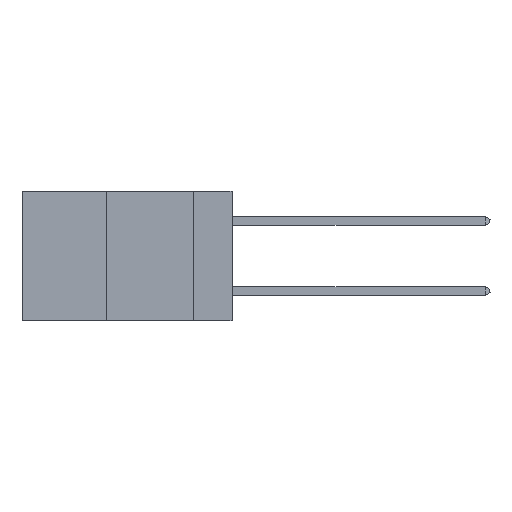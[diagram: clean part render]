
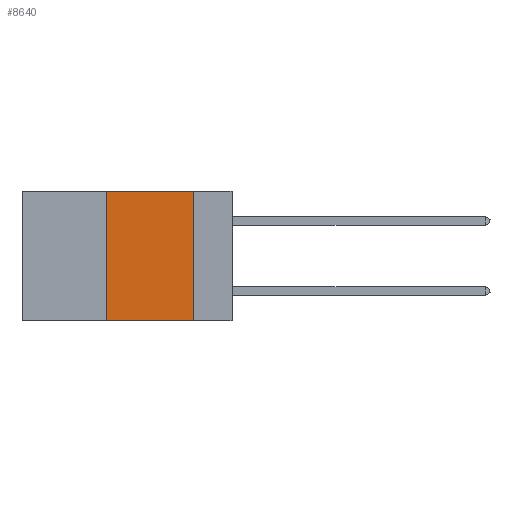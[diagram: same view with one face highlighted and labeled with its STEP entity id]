
A CAD part, left-side view. The second image highlights one B-rep face of the part: STEP entity #8640.
In plain terms, the highlighted planar face has unit normal (-1, 0, 0).
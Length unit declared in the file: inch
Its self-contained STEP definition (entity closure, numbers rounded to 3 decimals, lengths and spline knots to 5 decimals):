
#1943 = FACE_OUTER_BOUND ( 'NONE', #2229, .T. ) ;
#2229 = EDGE_LOOP ( 'NONE', ( #39148, #40176, #15780, #28841 ) ) ;
#3651 = LINE ( 'NONE', #20212, #40150 ) ;
#5818 = DIRECTION ( 'NONE',  ( 0., 0., -1. ) ) ;
#5874 = LINE ( 'NONE', #18531, #33836 ) ;
#6734 = EDGE_CURVE ( 'NONE', #27551, #7271, #3651, .T. ) ;
#7271 = VERTEX_POINT ( 'NONE', #43667 ) ;
#7871 = VECTOR ( 'NONE', #42710, 39.37008 ) ;
#8640 = ADVANCED_FACE ( 'NONE', ( #1943 ), #13028, .F. ) ;
#9150 = DIRECTION ( 'NONE',  ( 0., -1., 0. ) ) ;
#9687 = EDGE_CURVE ( 'NONE', #7271, #20230, #5874, .T. ) ;
#12099 = CARTESIAN_POINT ( 'NONE',  ( 0., 0.36, 0. ) ) ;
#13028 = PLANE ( 'NONE',  #21847 ) ;
#15780 = ORIENTED_EDGE ( 'NONE', *, *, #26651, .F. ) ;
#17183 = CARTESIAN_POINT ( 'NONE',  ( 0., 0.6, 0. ) ) ;
#18148 = LINE ( 'NONE', #45763, #7871 ) ;
#18531 = CARTESIAN_POINT ( 'NONE',  ( 0., 0.11, 0. ) ) ;
#20212 = CARTESIAN_POINT ( 'NONE',  ( 0., 0.6, 0. ) ) ;
#20230 = VERTEX_POINT ( 'NONE', #45911 ) ;
#21570 = LINE ( 'NONE', #32824, #31854 ) ;
#21847 = AXIS2_PLACEMENT_3D ( 'NONE', #17183, #27699, #5818 ) ;
#26651 = EDGE_CURVE ( 'NONE', #47073, #27551, #18148, .T. ) ;
#27551 = VERTEX_POINT ( 'NONE', #12099 ) ;
#27699 = DIRECTION ( 'NONE',  ( 1., 0., 0. ) ) ;
#28718 = DIRECTION ( 'NONE',  ( 0., -1., 0. ) ) ;
#28841 = ORIENTED_EDGE ( 'NONE', *, *, #30833, .T. ) ;
#29522 = DIRECTION ( 'NONE',  ( 0., 0., -1. ) ) ;
#30833 = EDGE_CURVE ( 'NONE', #47073, #20230, #21570, .T. ) ;
#31854 = VECTOR ( 'NONE', #28718, 39.37008 ) ;
#32824 = CARTESIAN_POINT ( 'NONE',  ( 0., 0.6, -0.37 ) ) ;
#33545 = CARTESIAN_POINT ( 'NONE',  ( 0., 0.36, -0.37 ) ) ;
#33836 = VECTOR ( 'NONE', #29522, 39.37008 ) ;
#39148 = ORIENTED_EDGE ( 'NONE', *, *, #9687, .F. ) ;
#40150 = VECTOR ( 'NONE', #9150, 39.37008 ) ;
#40176 = ORIENTED_EDGE ( 'NONE', *, *, #6734, .F. ) ;
#42710 = DIRECTION ( 'NONE',  ( 0., 0., 1. ) ) ;
#43667 = CARTESIAN_POINT ( 'NONE',  ( 0., 0.11, 0. ) ) ;
#45763 = CARTESIAN_POINT ( 'NONE',  ( 0., 0.36, 0. ) ) ;
#45911 = CARTESIAN_POINT ( 'NONE',  ( 0., 0.11, -0.37 ) ) ;
#47073 = VERTEX_POINT ( 'NONE', #33545 ) ;
